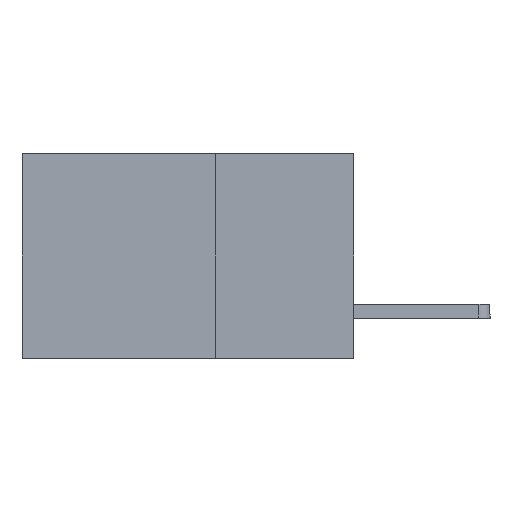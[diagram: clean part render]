
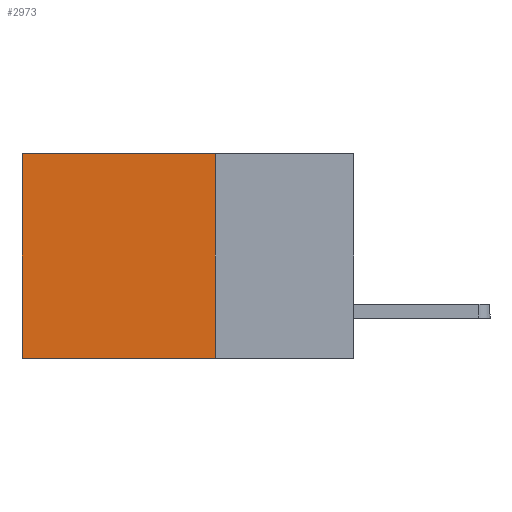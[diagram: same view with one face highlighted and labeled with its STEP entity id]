
A CAD part, left-side view. The second image highlights one B-rep face of the part: STEP entity #2973.
In plain terms, the highlighted planar face has unit normal (-1, 0, 0).
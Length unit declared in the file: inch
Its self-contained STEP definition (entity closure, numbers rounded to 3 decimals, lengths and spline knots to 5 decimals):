
#106 = EDGE_CURVE ( 'NONE', #6226, #3235, #5745, .T. ) ;
#213 = DIRECTION ( 'NONE',  ( 0., 0., -1. ) ) ;
#501 = LINE ( 'NONE', #6935, #7886 ) ;
#879 = VECTOR ( 'NONE', #4652, 39.37008 ) ;
#1403 = LINE ( 'NONE', #5542, #3154 ) ;
#1825 = CARTESIAN_POINT ( 'NONE',  ( 0.2875, 0.25, 0. ) ) ;
#1978 = ORIENTED_EDGE ( 'NONE', *, *, #2693, .F. ) ;
#2466 = FACE_OUTER_BOUND ( 'NONE', #4908, .T. ) ;
#2693 = EDGE_CURVE ( 'NONE', #3685, #6226, #501, .T. ) ;
#2911 = LINE ( 'NONE', #5931, #879 ) ;
#2973 = ADVANCED_FACE ( 'NONE', ( #2466 ), #8119, .F. ) ;
#2983 = CARTESIAN_POINT ( 'NONE',  ( 0.2875, 0.25, 0. ) ) ;
#3154 = VECTOR ( 'NONE', #6219, 39.37008 ) ;
#3235 = VERTEX_POINT ( 'NONE', #7170 ) ;
#3328 = ORIENTED_EDGE ( 'NONE', *, *, #8186, .T. ) ;
#3633 = VERTEX_POINT ( 'NONE', #8066 ) ;
#3685 = VERTEX_POINT ( 'NONE', #2983 ) ;
#3694 = CARTESIAN_POINT ( 'NONE',  ( 0.2875, 0.25, -0.37 ) ) ;
#3959 = VECTOR ( 'NONE', #7916, 39.37008 ) ;
#4124 = CARTESIAN_POINT ( 'NONE',  ( 0.2875, 0.25, -0.37 ) ) ;
#4652 = DIRECTION ( 'NONE',  ( 0., 1., 0. ) ) ;
#4908 = EDGE_LOOP ( 'NONE', ( #3328, #5834, #1978, #6671 ) ) ;
#4935 = AXIS2_PLACEMENT_3D ( 'NONE', #1825, #8259, #5298 ) ;
#5298 = DIRECTION ( 'NONE',  ( 0., 0., -1. ) ) ;
#5542 = CARTESIAN_POINT ( 'NONE',  ( 0.2875, 0.6, 0. ) ) ;
#5745 = LINE ( 'NONE', #4124, #3959 ) ;
#5834 = ORIENTED_EDGE ( 'NONE', *, *, #106, .F. ) ;
#5931 = CARTESIAN_POINT ( 'NONE',  ( 0.2875, 0.25, 0. ) ) ;
#6219 = DIRECTION ( 'NONE',  ( 0., 0., -1. ) ) ;
#6226 = VERTEX_POINT ( 'NONE', #3694 ) ;
#6671 = ORIENTED_EDGE ( 'NONE', *, *, #9120, .T. ) ;
#6935 = CARTESIAN_POINT ( 'NONE',  ( 0.2875, 0.25, 0. ) ) ;
#7170 = CARTESIAN_POINT ( 'NONE',  ( 0.2875, 0.6, -0.37 ) ) ;
#7886 = VECTOR ( 'NONE', #213, 39.37008 ) ;
#7916 = DIRECTION ( 'NONE',  ( 0., 1., 0. ) ) ;
#8066 = CARTESIAN_POINT ( 'NONE',  ( 0.2875, 0.6, 0. ) ) ;
#8119 = PLANE ( 'NONE',  #4935 ) ;
#8186 = EDGE_CURVE ( 'NONE', #3633, #3235, #1403, .T. ) ;
#8259 = DIRECTION ( 'NONE',  ( 1., 0., 0. ) ) ;
#9120 = EDGE_CURVE ( 'NONE', #3685, #3633, #2911, .T. ) ;
